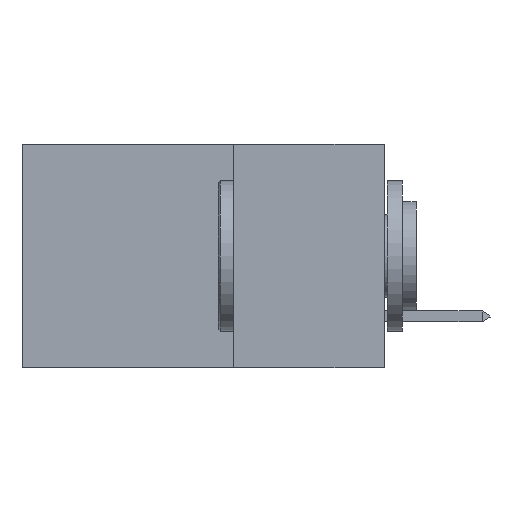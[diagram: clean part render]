
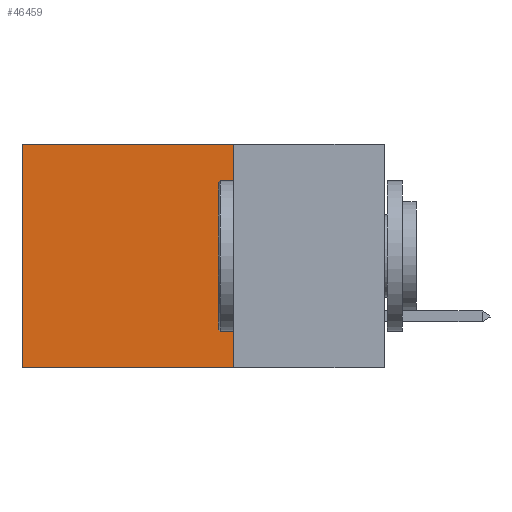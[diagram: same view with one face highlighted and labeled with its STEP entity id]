
A CAD part, left-side view. The second image highlights one B-rep face of the part: STEP entity #46459.
In plain terms, the highlighted planar face has unit normal (-1, 0, 0).
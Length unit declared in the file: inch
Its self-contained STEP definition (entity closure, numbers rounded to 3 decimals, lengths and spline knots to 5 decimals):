
#969 = DIRECTION ( 'NONE',  ( 0., 0., -1. ) ) ;
#1135 = LINE ( 'NONE', #13632, #19568 ) ;
#3480 = VECTOR ( 'NONE', #40279, 39.37008 ) ;
#4578 = ORIENTED_EDGE ( 'NONE', *, *, #11879, .F. ) ;
#7480 = VERTEX_POINT ( 'NONE', #8093 ) ;
#7924 = CARTESIAN_POINT ( 'NONE',  ( 0.2875, 0.25, 0. ) ) ;
#8093 = CARTESIAN_POINT ( 'NONE',  ( 0.2875, 0.25, 0. ) ) ;
#8692 = CARTESIAN_POINT ( 'NONE',  ( 0.2875, 0.25, -0.37 ) ) ;
#11852 = DIRECTION ( 'NONE',  ( 0., 1., 0. ) ) ;
#11879 = EDGE_CURVE ( 'NONE', #43866, #49136, #1135, .T. ) ;
#12265 = EDGE_CURVE ( 'NONE', #7480, #15071, #47795, .T. ) ;
#12480 = CARTESIAN_POINT ( 'NONE',  ( 0.2875, 0.6, 0. ) ) ;
#12988 = CARTESIAN_POINT ( 'NONE',  ( 0.2875, 0.6, -0.37 ) ) ;
#13632 = CARTESIAN_POINT ( 'NONE',  ( 0.2875, 0.25, -0.37 ) ) ;
#15071 = VERTEX_POINT ( 'NONE', #12480 ) ;
#15664 = ORIENTED_EDGE ( 'NONE', *, *, #21456, .T. ) ;
#15932 = CARTESIAN_POINT ( 'NONE',  ( 0.2875, 0.25, 0. ) ) ;
#18488 = DIRECTION ( 'NONE',  ( 0., 0., -1. ) ) ;
#19568 = VECTOR ( 'NONE', #21729, 39.37008 ) ;
#21456 = EDGE_CURVE ( 'NONE', #15071, #49136, #40929, .T. ) ;
#21729 = DIRECTION ( 'NONE',  ( 0., 1., 0. ) ) ;
#22297 = CARTESIAN_POINT ( 'NONE',  ( 0.2875, 0.25, 0. ) ) ;
#27560 = FACE_OUTER_BOUND ( 'NONE', #45773, .T. ) ;
#28573 = CARTESIAN_POINT ( 'NONE',  ( 0.2875, 0.6, 0. ) ) ;
#28711 = VECTOR ( 'NONE', #11852, 39.37008 ) ;
#30185 = DIRECTION ( 'NONE',  ( 1., 0., 0. ) ) ;
#32109 = AXIS2_PLACEMENT_3D ( 'NONE', #22297, #30185, #18488 ) ;
#35279 = ORIENTED_EDGE ( 'NONE', *, *, #12265, .T. ) ;
#36158 = VECTOR ( 'NONE', #969, 39.37008 ) ;
#38722 = ORIENTED_EDGE ( 'NONE', *, *, #48620, .F. ) ;
#40279 = DIRECTION ( 'NONE',  ( 0., 0., -1. ) ) ;
#40929 = LINE ( 'NONE', #28573, #3480 ) ;
#41655 = LINE ( 'NONE', #15932, #36158 ) ;
#43866 = VERTEX_POINT ( 'NONE', #8692 ) ;
#45302 = PLANE ( 'NONE',  #32109 ) ;
#45773 = EDGE_LOOP ( 'NONE', ( #15664, #4578, #38722, #35279 ) ) ;
#46459 = ADVANCED_FACE ( 'NONE', ( #27560 ), #45302, .F. ) ;
#47795 = LINE ( 'NONE', #7924, #28711 ) ;
#48620 = EDGE_CURVE ( 'NONE', #7480, #43866, #41655, .T. ) ;
#49136 = VERTEX_POINT ( 'NONE', #12988 ) ;
